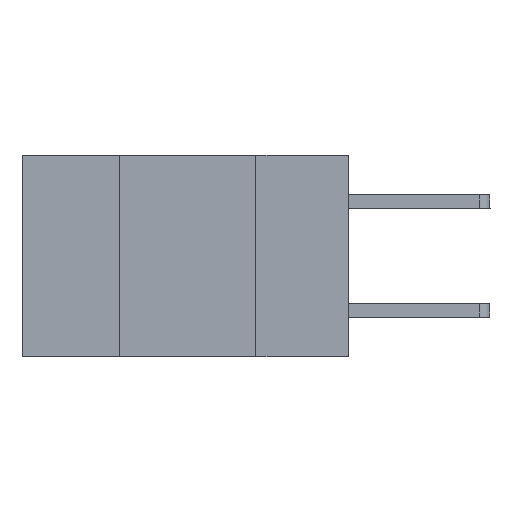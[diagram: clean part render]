
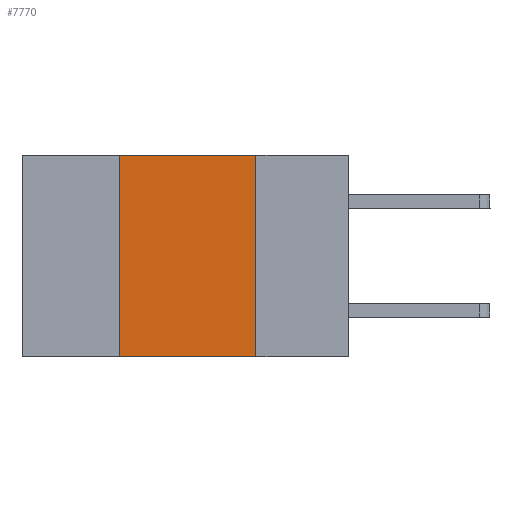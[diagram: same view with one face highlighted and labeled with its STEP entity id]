
A CAD part, left-side view. The second image highlights one B-rep face of the part: STEP entity #7770.
In plain terms, the highlighted planar face has unit normal (-1, 0, 0).
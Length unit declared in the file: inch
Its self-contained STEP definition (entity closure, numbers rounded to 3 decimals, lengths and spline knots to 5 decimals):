
#46 = DIRECTION ( 'NONE',  ( 0., -1., 0. ) ) ;
#667 = CARTESIAN_POINT ( 'NONE',  ( 0., 0.17, 0. ) ) ;
#804 = ORIENTED_EDGE ( 'NONE', *, *, #1800, .T. ) ;
#994 = CARTESIAN_POINT ( 'NONE',  ( 0., 0.42, -0.37 ) ) ;
#1395 = CARTESIAN_POINT ( 'NONE',  ( 0., 0.42, 0. ) ) ;
#1729 = ORIENTED_EDGE ( 'NONE', *, *, #5396, .F. ) ;
#1800 = EDGE_CURVE ( 'NONE', #9528, #2612, #3723, .T. ) ;
#1828 = VECTOR ( 'NONE', #6344, 39.37008 ) ;
#1877 = DIRECTION ( 'NONE',  ( 1., 0., 0. ) ) ;
#2046 = AXIS2_PLACEMENT_3D ( 'NONE', #3293, #1877, #4814 ) ;
#2057 = EDGE_CURVE ( 'NONE', #9528, #5435, #5575, .T. ) ;
#2126 = VECTOR ( 'NONE', #9772, 39.37008 ) ;
#2337 = DIRECTION ( 'NONE',  ( 0., 0., -1. ) ) ;
#2612 = VERTEX_POINT ( 'NONE', #2654 ) ;
#2654 = CARTESIAN_POINT ( 'NONE',  ( 0., 0.17, -0.37 ) ) ;
#3151 = VECTOR ( 'NONE', #2337, 39.37008 ) ;
#3293 = CARTESIAN_POINT ( 'NONE',  ( 0., 0.6, 0. ) ) ;
#3723 = LINE ( 'NONE', #6740, #2126 ) ;
#4132 = FACE_OUTER_BOUND ( 'NONE', #8217, .T. ) ;
#4571 = LINE ( 'NONE', #6815, #5291 ) ;
#4746 = ORIENTED_EDGE ( 'NONE', *, *, #8619, .F. ) ;
#4814 = DIRECTION ( 'NONE',  ( 0., 0., -1. ) ) ;
#5291 = VECTOR ( 'NONE', #46, 39.37008 ) ;
#5396 = EDGE_CURVE ( 'NONE', #5435, #6698, #4571, .T. ) ;
#5435 = VERTEX_POINT ( 'NONE', #1395 ) ;
#5575 = LINE ( 'NONE', #994, #1828 ) ;
#6139 = CARTESIAN_POINT ( 'NONE',  ( 0., 0.17, -0.37 ) ) ;
#6344 = DIRECTION ( 'NONE',  ( 0., 0., 1. ) ) ;
#6698 = VERTEX_POINT ( 'NONE', #667 ) ;
#6740 = CARTESIAN_POINT ( 'NONE',  ( 0., 0.6, -0.37 ) ) ;
#6815 = CARTESIAN_POINT ( 'NONE',  ( 0., 0.6, 0. ) ) ;
#7668 = LINE ( 'NONE', #6139, #3151 ) ;
#7770 = ADVANCED_FACE ( 'NONE', ( #4132 ), #8588, .F. ) ;
#8217 = EDGE_LOOP ( 'NONE', ( #4746, #1729, #9071, #804 ) ) ;
#8588 = PLANE ( 'NONE',  #2046 ) ;
#8619 = EDGE_CURVE ( 'NONE', #6698, #2612, #7668, .T. ) ;
#9071 = ORIENTED_EDGE ( 'NONE', *, *, #2057, .F. ) ;
#9278 = CARTESIAN_POINT ( 'NONE',  ( 0., 0.42, -0.37 ) ) ;
#9528 = VERTEX_POINT ( 'NONE', #9278 ) ;
#9772 = DIRECTION ( 'NONE',  ( 0., -1., 0. ) ) ;
